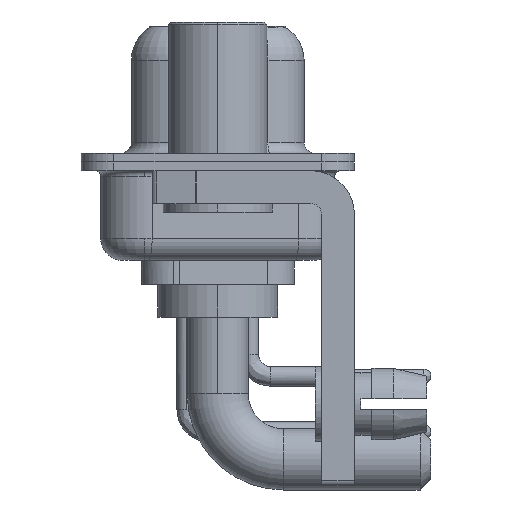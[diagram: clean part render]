
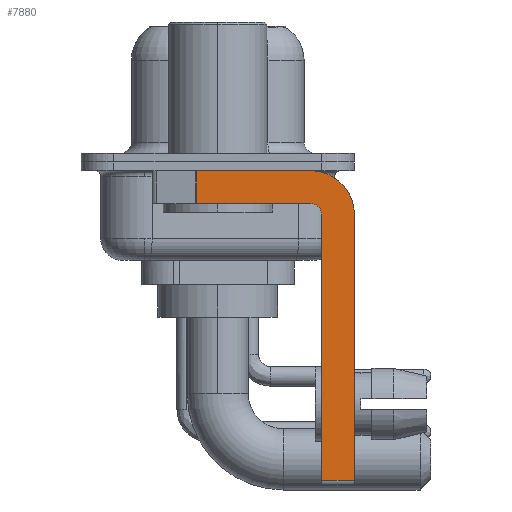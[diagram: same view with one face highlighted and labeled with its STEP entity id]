
A CAD part, left-side view. The second image highlights one B-rep face of the part: STEP entity #7880.
In plain terms, the highlighted planar face has unit normal (-1, 0, 0).
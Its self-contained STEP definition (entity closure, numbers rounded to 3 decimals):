
#773 = AXIS2_PLACEMENT_3D ( 'NONE', #21848, #20139, #11676 ) ;
#1045 = CIRCLE ( 'NONE', #11633, 2. ) ;
#1175 = VECTOR ( 'NONE', #6344, 1000. ) ;
#1593 = VERTEX_POINT ( 'NONE', #14198 ) ;
#2519 = CARTESIAN_POINT ( 'NONE',  ( -2.9, 0.978, -1.9 ) ) ;
#2783 = DIRECTION ( 'NONE',  ( 0., 0., -1. ) ) ;
#2856 = EDGE_CURVE ( 'NONE', #1593, #14778, #12874, .T. ) ;
#2937 = LINE ( 'NONE', #2519, #10296 ) ;
#3475 = AXIS2_PLACEMENT_3D ( 'NONE', #15129, #14903, #2783 ) ;
#4080 = CARTESIAN_POINT ( 'NONE',  ( -2.9, 0.978, -0.4 ) ) ;
#4117 = DIRECTION ( 'NONE',  ( 0., 1., 0. ) ) ;
#4548 = EDGE_CURVE ( 'NONE', #1593, #20438, #10744, .T. ) ;
#4618 = VERTEX_POINT ( 'NONE', #5705 ) ;
#5220 = EDGE_CURVE ( 'NONE', #11677, #10100, #5299, .T. ) ;
#5232 = CARTESIAN_POINT ( 'NONE',  ( -2.9, -4.25, -1.9 ) ) ;
#5299 = LINE ( 'NONE', #21406, #14693 ) ;
#5705 = CARTESIAN_POINT ( 'NONE',  ( -2.9, -6.25, -2.4 ) ) ;
#6262 = EDGE_CURVE ( 'NONE', #4618, #14778, #22514, .T. ) ;
#6344 = DIRECTION ( 'NONE',  ( 0., -1., 0. ) ) ;
#6847 = DIRECTION ( 'NONE',  ( 0., 0., -1. ) ) ;
#7084 = DIRECTION ( 'NONE',  ( 0., 0., 1. ) ) ;
#7437 = ORIENTED_EDGE ( 'NONE', *, *, #4548, .F. ) ;
#7693 = ORIENTED_EDGE ( 'NONE', *, *, #15985, .T. ) ;
#7880 = ADVANCED_FACE ( 'NONE', ( #14793 ), #11472, .F. ) ;
#8137 = CARTESIAN_POINT ( 'NONE',  ( -2.9, -4.75, -2.4 ) ) ;
#9288 = CARTESIAN_POINT ( 'NONE',  ( -2.9, 0.978, -1.9 ) ) ;
#9376 = ORIENTED_EDGE ( 'NONE', *, *, #5220, .F. ) ;
#9423 = VERTEX_POINT ( 'NONE', #9288 ) ;
#10100 = VERTEX_POINT ( 'NONE', #14979 ) ;
#10252 = ORIENTED_EDGE ( 'NONE', *, *, #2856, .T. ) ;
#10296 = VECTOR ( 'NONE', #17113, 1000. ) ;
#10340 = VECTOR ( 'NONE', #4117, 1000. ) ;
#10620 = CIRCLE ( 'NONE', #773, 0.5 ) ;
#10744 = LINE ( 'NONE', #21132, #21250 ) ;
#11472 = PLANE ( 'NONE',  #3475 ) ;
#11633 = AXIS2_PLACEMENT_3D ( 'NONE', #20543, #17014, #11957 ) ;
#11676 = DIRECTION ( 'NONE',  ( 0., 0., 1. ) ) ;
#11677 = VERTEX_POINT ( 'NONE', #4080 ) ;
#11957 = DIRECTION ( 'NONE',  ( 0., 0., -1. ) ) ;
#11976 = EDGE_CURVE ( 'NONE', #10100, #4618, #1045, .T. ) ;
#12874 = LINE ( 'NONE', #20183, #1175 ) ;
#14198 = CARTESIAN_POINT ( 'NONE',  ( -2.9, -4.75, -14.55 ) ) ;
#14335 = DIRECTION ( 'NONE',  ( 0., -1., 0. ) ) ;
#14693 = VECTOR ( 'NONE', #14335, 1000. ) ;
#14778 = VERTEX_POINT ( 'NONE', #20746 ) ;
#14793 = FACE_OUTER_BOUND ( 'NONE', #21508, .T. ) ;
#14903 = DIRECTION ( 'NONE',  ( 1., 0., 0. ) ) ;
#14979 = CARTESIAN_POINT ( 'NONE',  ( -2.9, -4.25, -0.4 ) ) ;
#15129 = CARTESIAN_POINT ( 'NONE',  ( -2.9, -4.25, -2.4 ) ) ;
#15544 = EDGE_CURVE ( 'NONE', #20438, #22452, #10620, .T. ) ;
#15824 = LINE ( 'NONE', #16606, #10340 ) ;
#15985 = EDGE_CURVE ( 'NONE', #11677, #9423, #2937, .T. ) ;
#16438 = ORIENTED_EDGE ( 'NONE', *, *, #6262, .F. ) ;
#16606 = CARTESIAN_POINT ( 'NONE',  ( -2.9, -4.25, -1.9 ) ) ;
#16861 = ORIENTED_EDGE ( 'NONE', *, *, #15544, .F. ) ;
#17014 = DIRECTION ( 'NONE',  ( 1., 0., 0. ) ) ;
#17113 = DIRECTION ( 'NONE',  ( 0., 0., -1. ) ) ;
#17478 = CARTESIAN_POINT ( 'NONE',  ( -2.9, -6.25, -2.4 ) ) ;
#18576 = EDGE_CURVE ( 'NONE', #22452, #9423, #15824, .T. ) ;
#18776 = VECTOR ( 'NONE', #6847, 1000. ) ;
#18962 = ORIENTED_EDGE ( 'NONE', *, *, #11976, .F. ) ;
#20139 = DIRECTION ( 'NONE',  ( -1., 0., 0. ) ) ;
#20183 = CARTESIAN_POINT ( 'NONE',  ( -2.9, -4.25, -14.55 ) ) ;
#20438 = VERTEX_POINT ( 'NONE', #8137 ) ;
#20543 = CARTESIAN_POINT ( 'NONE',  ( -2.9, -4.25, -2.4 ) ) ;
#20746 = CARTESIAN_POINT ( 'NONE',  ( -2.9, -6.25, -14.55 ) ) ;
#21132 = CARTESIAN_POINT ( 'NONE',  ( -2.9, -4.75, -14.8 ) ) ;
#21250 = VECTOR ( 'NONE', #7084, 1000. ) ;
#21406 = CARTESIAN_POINT ( 'NONE',  ( -2.9, 3., -0.4 ) ) ;
#21508 = EDGE_LOOP ( 'NONE', ( #9376, #7693, #21877, #16861, #7437, #10252, #16438, #18962 ) ) ;
#21848 = CARTESIAN_POINT ( 'NONE',  ( -2.9, -4.25, -2.4 ) ) ;
#21877 = ORIENTED_EDGE ( 'NONE', *, *, #18576, .F. ) ;
#22452 = VERTEX_POINT ( 'NONE', #5232 ) ;
#22514 = LINE ( 'NONE', #17478, #18776 ) ;
